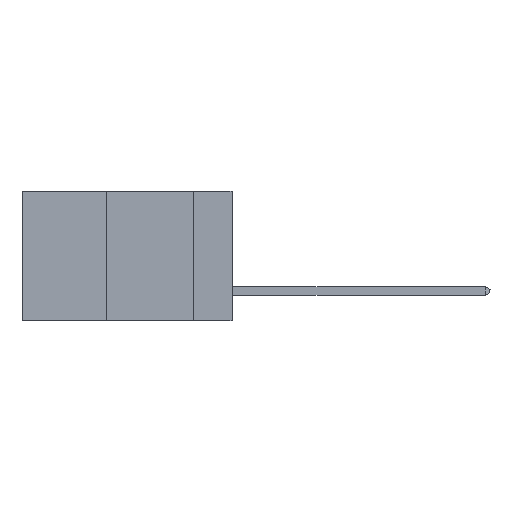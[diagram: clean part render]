
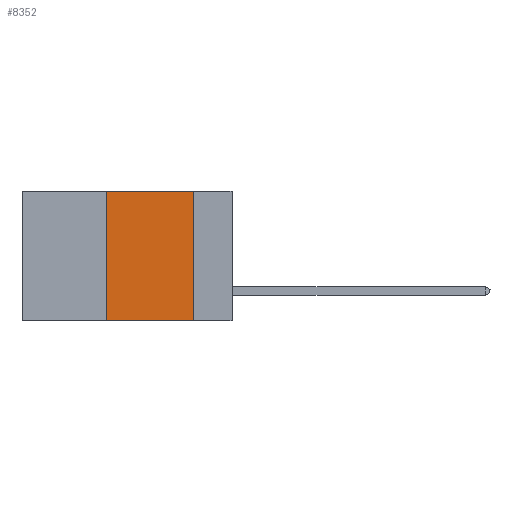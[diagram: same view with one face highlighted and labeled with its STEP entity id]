
A CAD part, left-side view. The second image highlights one B-rep face of the part: STEP entity #8352.
In plain terms, the highlighted planar face has unit normal (-1, 0, 0).
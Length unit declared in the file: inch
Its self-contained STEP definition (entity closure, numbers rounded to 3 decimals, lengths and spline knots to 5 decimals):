
#440 = ORIENTED_EDGE ( 'NONE', *, *, #10354, .F. ) ;
#650 = LINE ( 'NONE', #10402, #7395 ) ;
#728 = DIRECTION ( 'NONE',  ( 0., -1., 0. ) ) ;
#1631 = LINE ( 'NONE', #10718, #10284 ) ;
#1918 = VECTOR ( 'NONE', #9830, 39.37008 ) ;
#3240 = CARTESIAN_POINT ( 'NONE',  ( 0., 0.6, 0. ) ) ;
#3610 = CARTESIAN_POINT ( 'NONE',  ( 0., 0.36, 0. ) ) ;
#3691 = EDGE_LOOP ( 'NONE', ( #440, #10566, #5029, #6685 ) ) ;
#3864 = AXIS2_PLACEMENT_3D ( 'NONE', #3240, #9339, #5817 ) ;
#4763 = VERTEX_POINT ( 'NONE', #5445 ) ;
#4772 = VERTEX_POINT ( 'NONE', #6570 ) ;
#4904 = VECTOR ( 'NONE', #7739, 39.37008 ) ;
#5029 = ORIENTED_EDGE ( 'NONE', *, *, #8959, .F. ) ;
#5080 = CARTESIAN_POINT ( 'NONE',  ( 0., 0.11, 0. ) ) ;
#5445 = CARTESIAN_POINT ( 'NONE',  ( 0., 0.36, 0. ) ) ;
#5817 = DIRECTION ( 'NONE',  ( 0., 0., -1. ) ) ;
#5887 = LINE ( 'NONE', #3610, #1918 ) ;
#5904 = FACE_OUTER_BOUND ( 'NONE', #3691, .T. ) ;
#6426 = VERTEX_POINT ( 'NONE', #8016 ) ;
#6570 = CARTESIAN_POINT ( 'NONE',  ( 0., 0.36, -0.37 ) ) ;
#6639 = CARTESIAN_POINT ( 'NONE',  ( 0., 0.11, 0. ) ) ;
#6685 = ORIENTED_EDGE ( 'NONE', *, *, #10326, .T. ) ;
#7203 = VERTEX_POINT ( 'NONE', #6639 ) ;
#7395 = VECTOR ( 'NONE', #728, 39.37008 ) ;
#7739 = DIRECTION ( 'NONE',  ( 0., 0., -1. ) ) ;
#8009 = DIRECTION ( 'NONE',  ( 0., -1., 0. ) ) ;
#8016 = CARTESIAN_POINT ( 'NONE',  ( 0., 0.11, -0.37 ) ) ;
#8343 = LINE ( 'NONE', #5080, #4904 ) ;
#8352 = ADVANCED_FACE ( 'NONE', ( #5904 ), #9265, .F. ) ;
#8959 = EDGE_CURVE ( 'NONE', #4772, #4763, #5887, .T. ) ;
#9265 = PLANE ( 'NONE',  #3864 ) ;
#9339 = DIRECTION ( 'NONE',  ( 1., 0., 0. ) ) ;
#9592 = EDGE_CURVE ( 'NONE', #4763, #7203, #1631, .T. ) ;
#9830 = DIRECTION ( 'NONE',  ( 0., 0., 1. ) ) ;
#10284 = VECTOR ( 'NONE', #8009, 39.37008 ) ;
#10326 = EDGE_CURVE ( 'NONE', #4772, #6426, #650, .T. ) ;
#10354 = EDGE_CURVE ( 'NONE', #7203, #6426, #8343, .T. ) ;
#10402 = CARTESIAN_POINT ( 'NONE',  ( 0., 0.6, -0.37 ) ) ;
#10566 = ORIENTED_EDGE ( 'NONE', *, *, #9592, .F. ) ;
#10718 = CARTESIAN_POINT ( 'NONE',  ( 0., 0.6, 0. ) ) ;
